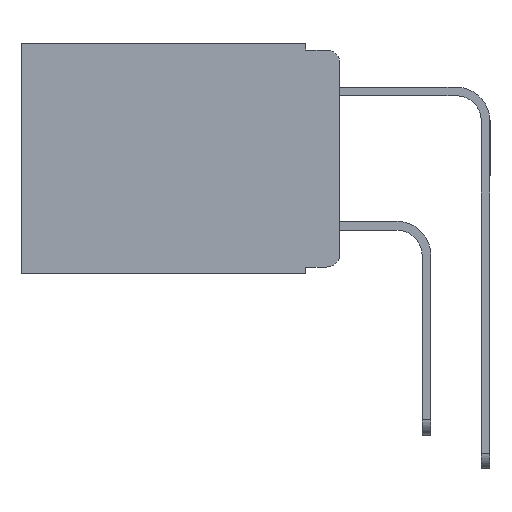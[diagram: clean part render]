
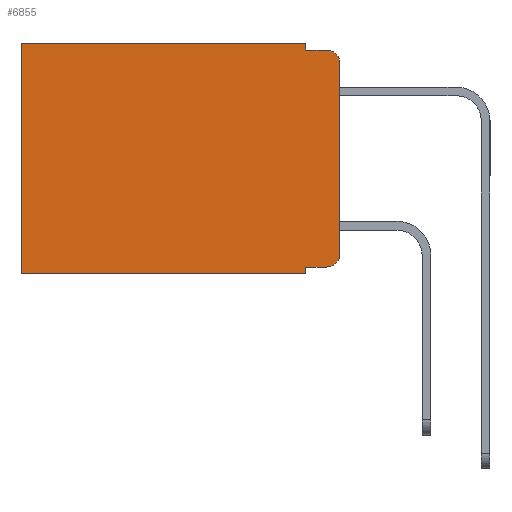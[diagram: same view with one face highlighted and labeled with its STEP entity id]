
A CAD part, left-side view. The second image highlights one B-rep face of the part: STEP entity #6855.
In plain terms, the highlighted planar face has unit normal (-1, 0, 0).
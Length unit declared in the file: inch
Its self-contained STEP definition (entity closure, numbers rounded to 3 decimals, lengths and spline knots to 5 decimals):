
#2 = CARTESIAN_POINT ( 'NONE',  ( 0.298, 0.051, -0.343 ) ) ;
#56 = VERTEX_POINT ( 'NONE', #8681 ) ;
#143 = DIRECTION ( 'NONE',  ( 0., 0., -1. ) ) ;
#473 = VERTEX_POINT ( 'NONE', #8621 ) ;
#783 = VERTEX_POINT ( 'NONE', #11148 ) ;
#948 = ORIENTED_EDGE ( 'NONE', *, *, #1694, .T. ) ;
#984 = ORIENTED_EDGE ( 'NONE', *, *, #4727, .T. ) ;
#1185 = VECTOR ( 'NONE', #11927, 39.37008 ) ;
#1210 = EDGE_CURVE ( 'NONE', #4151, #473, #7774, .T. ) ;
#1494 = AXIS2_PLACEMENT_3D ( 'NONE', #5914, #10456, #4634 ) ;
#1502 = CARTESIAN_POINT ( 'NONE',  ( 0.298, 0.02, -0.313 ) ) ;
#1694 = EDGE_CURVE ( 'NONE', #5562, #783, #1970, .T. ) ;
#1804 = VERTEX_POINT ( 'NONE', #12868 ) ;
#1970 = CIRCLE ( 'NONE', #4268, 0.02 ) ;
#1987 = VECTOR ( 'NONE', #8855, 39.37008 ) ;
#2053 = CARTESIAN_POINT ( 'NONE',  ( 0.298, 0., 0. ) ) ;
#2462 = LINE ( 'NONE', #7952, #10237 ) ;
#2603 = DIRECTION ( 'NONE',  ( 0., 0., -1. ) ) ;
#2707 = CARTESIAN_POINT ( 'NONE',  ( 0.298, 0.473, 0. ) ) ;
#2738 = ORIENTED_EDGE ( 'NONE', *, *, #6233, .T. ) ;
#2953 = EDGE_CURVE ( 'NONE', #12278, #783, #2462, .T. ) ;
#2971 = ORIENTED_EDGE ( 'NONE', *, *, #1210, .T. ) ;
#3344 = CARTESIAN_POINT ( 'NONE',  ( 0.298, 0., -0.343 ) ) ;
#3383 = DIRECTION ( 'NONE',  ( 0., 0., -1. ) ) ;
#3487 = ORIENTED_EDGE ( 'NONE', *, *, #9509, .T. ) ;
#3548 = VECTOR ( 'NONE', #143, 39.37008 ) ;
#3704 = LINE ( 'NONE', #11050, #6088 ) ;
#3985 = VECTOR ( 'NONE', #10035, 39.37008 ) ;
#4048 = EDGE_CURVE ( 'NONE', #4447, #5457, #3704, .T. ) ;
#4151 = VERTEX_POINT ( 'NONE', #2707 ) ;
#4268 = AXIS2_PLACEMENT_3D ( 'NONE', #9005, #12216, #6552 ) ;
#4397 = CARTESIAN_POINT ( 'NONE',  ( 0.298, 0.051, 0. ) ) ;
#4447 = VERTEX_POINT ( 'NONE', #6964 ) ;
#4634 = DIRECTION ( 'NONE',  ( 0., 0., -1. ) ) ;
#4727 = EDGE_CURVE ( 'NONE', #4447, #5282, #6077, .T. ) ;
#5120 = ORIENTED_EDGE ( 'NONE', *, *, #11649, .F. ) ;
#5282 = VERTEX_POINT ( 'NONE', #5424 ) ;
#5424 = CARTESIAN_POINT ( 'NONE',  ( 0.298, 0.02, -0.333 ) ) ;
#5457 = VERTEX_POINT ( 'NONE', #2 ) ;
#5562 = VERTEX_POINT ( 'NONE', #12455 ) ;
#5914 = CARTESIAN_POINT ( 'NONE',  ( 0.298, 0., 0. ) ) ;
#6077 = LINE ( 'NONE', #10130, #10796 ) ;
#6084 = EDGE_CURVE ( 'NONE', #5457, #473, #11910, .T. ) ;
#6088 = VECTOR ( 'NONE', #3383, 39.37008 ) ;
#6233 = EDGE_CURVE ( 'NONE', #1804, #4151, #12939, .T. ) ;
#6311 = CARTESIAN_POINT ( 'NONE',  ( 0.298, 0.473, 0. ) ) ;
#6552 = DIRECTION ( 'NONE',  ( 0., 0., -1. ) ) ;
#6855 = ADVANCED_FACE ( 'NONE', ( #9375 ), #6983, .F. ) ;
#6964 = CARTESIAN_POINT ( 'NONE',  ( 0.298, 0.051, -0.333 ) ) ;
#6980 = DIRECTION ( 'NONE',  ( 0., -1., 0. ) ) ;
#6983 = PLANE ( 'NONE',  #1494 ) ;
#7415 = EDGE_LOOP ( 'NONE', ( #12638, #948, #12438, #5120, #2738, #2971, #8881, #7563, #984, #3487 ) ) ;
#7563 = ORIENTED_EDGE ( 'NONE', *, *, #4048, .F. ) ;
#7774 = LINE ( 'NONE', #6311, #1987 ) ;
#7952 = CARTESIAN_POINT ( 'NONE',  ( 0.298, 0.051, -0.01 ) ) ;
#8621 = CARTESIAN_POINT ( 'NONE',  ( 0.298, 0.473, -0.343 ) ) ;
#8681 = CARTESIAN_POINT ( 'NONE',  ( 0.298, 0., -0.313 ) ) ;
#8704 = DIRECTION ( 'NONE',  ( -1., 0., 0. ) ) ;
#8855 = DIRECTION ( 'NONE',  ( 0., 0., -1. ) ) ;
#8881 = ORIENTED_EDGE ( 'NONE', *, *, #6084, .F. ) ;
#9005 = CARTESIAN_POINT ( 'NONE',  ( 0.298, 0.02, -0.03 ) ) ;
#9107 = LINE ( 'NONE', #11002, #1185 ) ;
#9375 = FACE_OUTER_BOUND ( 'NONE', #7415, .T. ) ;
#9509 = EDGE_CURVE ( 'NONE', #5282, #56, #12143, .T. ) ;
#9633 = DIRECTION ( 'NONE',  ( 0., 1., 0. ) ) ;
#9724 = AXIS2_PLACEMENT_3D ( 'NONE', #1502, #8704, #2603 ) ;
#10035 = DIRECTION ( 'NONE',  ( 0., 1., 0. ) ) ;
#10130 = CARTESIAN_POINT ( 'NONE',  ( 0.298, 0.051, -0.333 ) ) ;
#10237 = VECTOR ( 'NONE', #6980, 39.37008 ) ;
#10456 = DIRECTION ( 'NONE',  ( 1., 0., 0. ) ) ;
#10796 = VECTOR ( 'NONE', #10803, 39.37008 ) ;
#10803 = DIRECTION ( 'NONE',  ( 0., -1., 0. ) ) ;
#11002 = CARTESIAN_POINT ( 'NONE',  ( 0.298, 0., 0. ) ) ;
#11050 = CARTESIAN_POINT ( 'NONE',  ( 0.298, 0.051, 0. ) ) ;
#11148 = CARTESIAN_POINT ( 'NONE',  ( 0.298, 0.02, -0.01 ) ) ;
#11172 = CARTESIAN_POINT ( 'NONE',  ( 0.298, 0.051, -0.01 ) ) ;
#11529 = LINE ( 'NONE', #4397, #3548 ) ;
#11649 = EDGE_CURVE ( 'NONE', #1804, #12278, #11529, .T. ) ;
#11910 = LINE ( 'NONE', #3344, #3985 ) ;
#11927 = DIRECTION ( 'NONE',  ( 0., 0., -1. ) ) ;
#12143 = CIRCLE ( 'NONE', #9724, 0.02 ) ;
#12216 = DIRECTION ( 'NONE',  ( -1., 0., 0. ) ) ;
#12278 = VERTEX_POINT ( 'NONE', #11172 ) ;
#12438 = ORIENTED_EDGE ( 'NONE', *, *, #2953, .F. ) ;
#12455 = CARTESIAN_POINT ( 'NONE',  ( 0.298, 0., -0.03 ) ) ;
#12638 = ORIENTED_EDGE ( 'NONE', *, *, #13057, .F. ) ;
#12640 = VECTOR ( 'NONE', #9633, 39.37008 ) ;
#12868 = CARTESIAN_POINT ( 'NONE',  ( 0.298, 0.051, 0. ) ) ;
#12939 = LINE ( 'NONE', #2053, #12640 ) ;
#13057 = EDGE_CURVE ( 'NONE', #5562, #56, #9107, .T. ) ;
